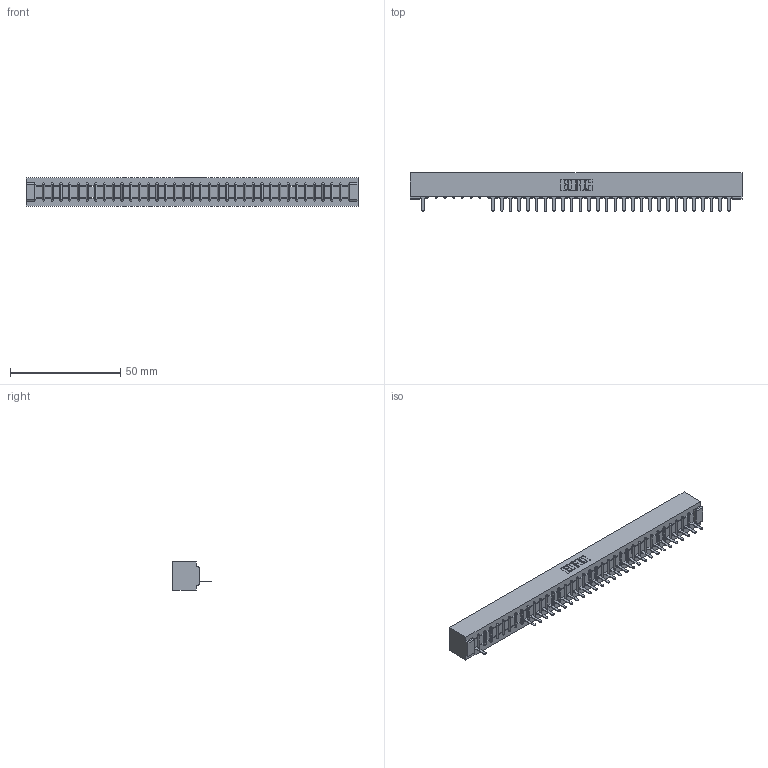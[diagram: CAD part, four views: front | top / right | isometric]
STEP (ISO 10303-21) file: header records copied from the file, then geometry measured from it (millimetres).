
FILE_DESCRIPTION (( 'STEP AP203' ), '1' );
FILE_NAME ('307-036-525-101.STEP', '2018-08-05T07:49:31', ( '' ), ( '' ), 'SwSTEP 2.0', 'SolidWorks 2016', '' );
FILE_SCHEMA (( 'CONFIG_CONTROL_DESIGN' ));
Length unit declared in the file: inch
Products named in the file (3): 307 Part_No Mounting Lugs; 307-290-001_525; 307-036-525-101
Assembly tree (30 placements, depth 2):
  307-036-525-101
    307 Part_No Mounting Lugs
    307-290-001_525  x29
Bounding box: 150.52 x 17.42 x 12.7 mm (x, y, z)
Volume: 15976.9 mm3; surface area: 16142.5 mm2
Topology: 30 solids, 30 shells, 1911 faces, 5445 edges, 3490 vertices
Faces by surface type: plane 1223, cylinder 614, sphere 74
Entity records: 31068 total; most frequent: CARTESIAN_POINT 5261, ORIENTED_EDGE 5254, DIRECTION 5111, EDGE_CURVE 2627, VECTOR 2015, LINE 2015, VERTEX_POINT 1698, AXIS2_PLACEMENT_3D 1548
